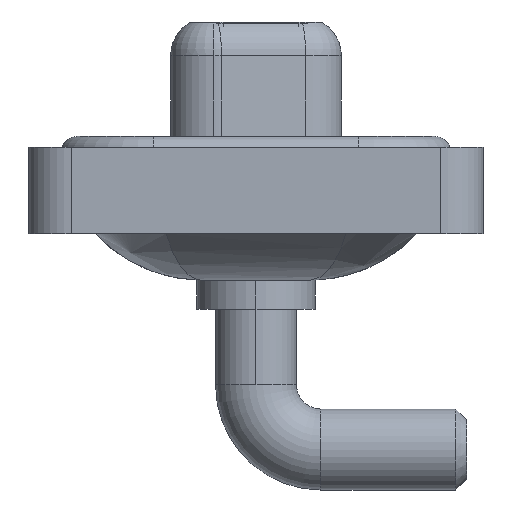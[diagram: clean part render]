
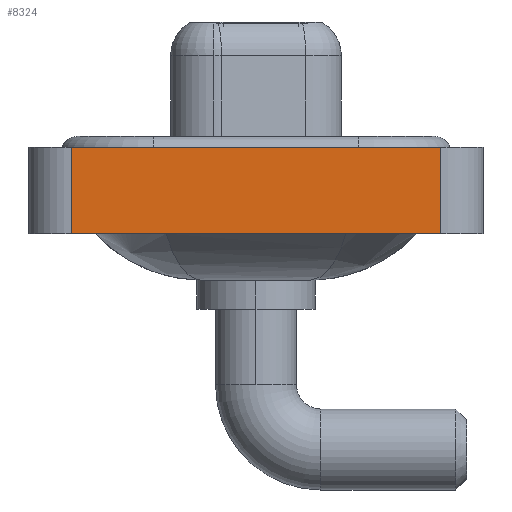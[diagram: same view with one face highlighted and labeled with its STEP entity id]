
A CAD part, left-side view. The second image highlights one B-rep face of the part: STEP entity #8324.
In plain terms, the highlighted planar face has unit normal (-1, 0, 0).
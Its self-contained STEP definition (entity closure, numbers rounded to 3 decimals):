
#799 = CARTESIAN_POINT ( 'NONE',  ( -7.3, -8.55, -3.6 ) ) ;
#883 = EDGE_CURVE ( 'NONE', #6363, #10297, #5913, .T. ) ;
#1394 = LINE ( 'NONE', #10422, #9134 ) ;
#1402 = VERTEX_POINT ( 'NONE', #6404 ) ;
#1568 = ORIENTED_EDGE ( 'NONE', *, *, #2592, .F. ) ;
#2592 = EDGE_CURVE ( 'NONE', #1402, #3265, #11110, .T. ) ;
#2969 = VECTOR ( 'NONE', #7190, 1000. ) ;
#2979 = EDGE_CURVE ( 'NONE', #6363, #1402, #1394, .T. ) ;
#3265 = VERTEX_POINT ( 'NONE', #4922 ) ;
#4245 = ORIENTED_EDGE ( 'NONE', *, *, #883, .T. ) ;
#4562 = CARTESIAN_POINT ( 'NONE',  ( -7.3, 8.55, -3.6 ) ) ;
#4599 = CARTESIAN_POINT ( 'NONE',  ( -7.3, -8.55, -3.6 ) ) ;
#4842 = DIRECTION ( 'NONE',  ( 0., 0., 1. ) ) ;
#4922 = CARTESIAN_POINT ( 'NONE',  ( -7.3, -8.55, 0.4 ) ) ;
#4925 = ORIENTED_EDGE ( 'NONE', *, *, #2979, .F. ) ;
#5913 = LINE ( 'NONE', #10852, #6438 ) ;
#6363 = VERTEX_POINT ( 'NONE', #4562 ) ;
#6404 = CARTESIAN_POINT ( 'NONE',  ( -7.3, 8.55, 0.4 ) ) ;
#6438 = VECTOR ( 'NONE', #13230, 1000. ) ;
#7190 = DIRECTION ( 'NONE',  ( 0., 0., 1. ) ) ;
#7459 = DIRECTION ( 'NONE',  ( 0., 0., 1. ) ) ;
#8324 = ADVANCED_FACE ( 'NONE', ( #10914 ), #8496, .T. ) ;
#8424 = AXIS2_PLACEMENT_3D ( 'NONE', #13373, #15872, #4842 ) ;
#8496 = PLANE ( 'NONE',  #8424 ) ;
#9134 = VECTOR ( 'NONE', #7459, 1000. ) ;
#10297 = VERTEX_POINT ( 'NONE', #799 ) ;
#10422 = CARTESIAN_POINT ( 'NONE',  ( -7.3, 8.55, -3.6 ) ) ;
#10756 = LINE ( 'NONE', #4599, #2969 ) ;
#10852 = CARTESIAN_POINT ( 'NONE',  ( -7.3, -8.55, -3.6 ) ) ;
#10914 = FACE_OUTER_BOUND ( 'NONE', #12691, .T. ) ;
#11110 = LINE ( 'NONE', #13409, #15771 ) ;
#11552 = ORIENTED_EDGE ( 'NONE', *, *, #15638, .T. ) ;
#12691 = EDGE_LOOP ( 'NONE', ( #11552, #1568, #4925, #4245 ) ) ;
#13230 = DIRECTION ( 'NONE',  ( 0., -1., 0. ) ) ;
#13373 = CARTESIAN_POINT ( 'NONE',  ( -7.3, -8.55, -3.6 ) ) ;
#13409 = CARTESIAN_POINT ( 'NONE',  ( -7.3, -8.55, 0.4 ) ) ;
#15006 = DIRECTION ( 'NONE',  ( 0., -1., 0. ) ) ;
#15638 = EDGE_CURVE ( 'NONE', #10297, #3265, #10756, .T. ) ;
#15771 = VECTOR ( 'NONE', #15006, 1000. ) ;
#15872 = DIRECTION ( 'NONE',  ( -1., 0., 0. ) ) ;
